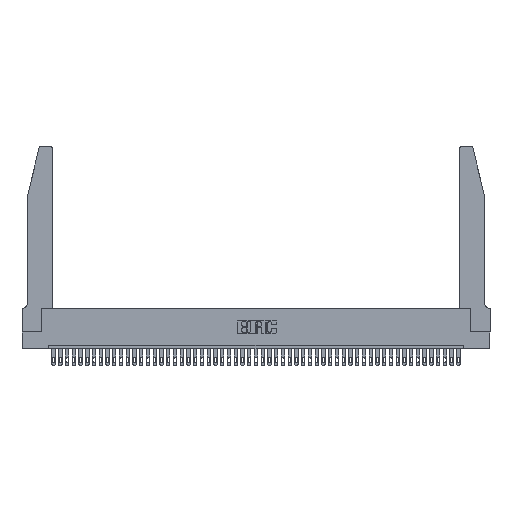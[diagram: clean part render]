
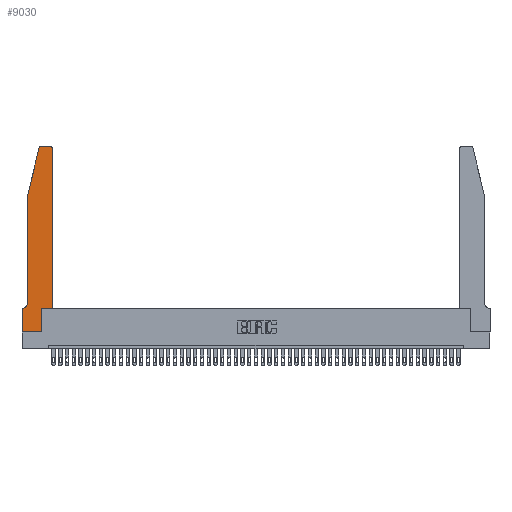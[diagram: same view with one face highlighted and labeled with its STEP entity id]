
A CAD part, top view. The second image highlights one B-rep face of the part: STEP entity #9030.
In plain terms, the highlighted planar face has unit normal (0, 0, 1).
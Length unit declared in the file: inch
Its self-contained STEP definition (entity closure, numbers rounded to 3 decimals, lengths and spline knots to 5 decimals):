
#95 = VERTEX_POINT ( 'NONE', #7106 ) ;
#144 = AXIS2_PLACEMENT_3D ( 'NONE', #27941, #35610, #2366 ) ;
#170 = ORIENTED_EDGE ( 'NONE', *, *, #24348, .T. ) ;
#1608 = DIRECTION ( 'NONE',  ( 0., 1., 0. ) ) ;
#2128 = CARTESIAN_POINT ( 'NONE',  ( 0.4205, 2.75, 0.37 ) ) ;
#2366 = DIRECTION ( 'NONE',  ( 1., 0., 0. ) ) ;
#3144 = VERTEX_POINT ( 'NONE', #28241 ) ;
#4175 = ORIENTED_EDGE ( 'NONE', *, *, #23835, .T. ) ;
#4460 = DIRECTION ( 'NONE',  ( -1., 0., 0. ) ) ;
#4820 = VERTEX_POINT ( 'NONE', #42210 ) ;
#4945 = VECTOR ( 'NONE', #26422, 39.37008 ) ;
#5229 = ORIENTED_EDGE ( 'NONE', *, *, #10144, .T. ) ;
#5287 = EDGE_CURVE ( 'NONE', #4820, #25033, #38751, .T. ) ;
#6729 = ORIENTED_EDGE ( 'NONE', *, *, #9586, .T. ) ;
#7106 = CARTESIAN_POINT ( 'NONE',  ( 0., 0.35, 0.37 ) ) ;
#7374 = LINE ( 'NONE', #19975, #15328 ) ;
#7543 = CIRCLE ( 'NONE', #144, 0.03 ) ;
#9030 = ADVANCED_FACE ( 'NONE', ( #33264 ), #16966, .T. ) ;
#9040 = DIRECTION ( 'NONE',  ( 1., 0., 0. ) ) ;
#9586 = EDGE_CURVE ( 'NONE', #3144, #27715, #7374, .T. ) ;
#10144 = EDGE_CURVE ( 'NONE', #19542, #3144, #37966, .T. ) ;
#10581 = CARTESIAN_POINT ( 'NONE',  ( 0.0755, 0.42, 0.37 ) ) ;
#11429 = VECTOR ( 'NONE', #36887, 39.37008 ) ;
#11593 = EDGE_CURVE ( 'NONE', #41714, #36071, #11748, .T. ) ;
#11667 = EDGE_CURVE ( 'NONE', #95, #19542, #26233, .T. ) ;
#11748 = LINE ( 'NONE', #12568, #47234 ) ;
#12568 = CARTESIAN_POINT ( 'NONE',  ( 0.4505, 0.35, 0.37 ) ) ;
#13299 = LINE ( 'NONE', #22866, #24337 ) ;
#13457 = DIRECTION ( 'NONE',  ( 1., 0., 0. ) ) ;
#13669 = CARTESIAN_POINT ( 'NONE',  ( 0.4505, 0.35, 0.37 ) ) ;
#13949 = EDGE_CURVE ( 'NONE', #34586, #14056, #14427, .T. ) ;
#14056 = VERTEX_POINT ( 'NONE', #46454 ) ;
#14427 = CIRCLE ( 'NONE', #47352, 0.07 ) ;
#14508 = CARTESIAN_POINT ( 'NONE',  ( 0.0055, 0.42, 0.37 ) ) ;
#14633 = VECTOR ( 'NONE', #15605, 39.37008 ) ;
#15246 = CARTESIAN_POINT ( 'NONE',  ( 0.0755, 2., 0.37 ) ) ;
#15328 = VECTOR ( 'NONE', #42264, 39.37008 ) ;
#15486 = CIRCLE ( 'NONE', #35171, 0.03 ) ;
#15596 = ORIENTED_EDGE ( 'NONE', *, *, #15885, .T. ) ;
#15605 = DIRECTION ( 'NONE',  ( 0., -1., 0. ) ) ;
#15843 = CARTESIAN_POINT ( 'NONE',  ( 0.4505, 2.72, 0.37 ) ) ;
#15885 = EDGE_CURVE ( 'NONE', #30623, #24158, #19601, .T. ) ;
#16187 = EDGE_CURVE ( 'NONE', #36071, #30623, #7543, .T. ) ;
#16415 = DIRECTION ( 'NONE',  ( -1., 0., 0. ) ) ;
#16966 = PLANE ( 'NONE',  #29522 ) ;
#18651 = DIRECTION ( 'NONE',  ( 0., 0., -1. ) ) ;
#19542 = VERTEX_POINT ( 'NONE', #23255 ) ;
#19601 = LINE ( 'NONE', #46045, #45235 ) ;
#19710 = ORIENTED_EDGE ( 'NONE', *, *, #32613, .T. ) ;
#19975 = CARTESIAN_POINT ( 'NONE',  ( 0.2865, 0.35, 0.37 ) ) ;
#20519 = ORIENTED_EDGE ( 'NONE', *, *, #5287, .T. ) ;
#20702 = CARTESIAN_POINT ( 'NONE',  ( 0., 0.35, 0.37 ) ) ;
#21926 = ORIENTED_EDGE ( 'NONE', *, *, #13949, .T. ) ;
#22655 = DIRECTION ( 'NONE',  ( 0., 0., 1. ) ) ;
#22698 = ORIENTED_EDGE ( 'NONE', *, *, #16187, .T. ) ;
#22866 = CARTESIAN_POINT ( 'NONE',  ( 0.0755, 0.35, 0.37 ) ) ;
#23255 = CARTESIAN_POINT ( 'NONE',  ( 0., 0., 0.37 ) ) ;
#23770 = CARTESIAN_POINT ( 'NONE',  ( 0., 0., 0.37 ) ) ;
#23835 = EDGE_CURVE ( 'NONE', #14056, #95, #13299, .T. ) ;
#24158 = VERTEX_POINT ( 'NONE', #37510 ) ;
#24337 = VECTOR ( 'NONE', #4460, 39.37008 ) ;
#24348 = EDGE_CURVE ( 'NONE', #24158, #4820, #15486, .T. ) ;
#24437 = CARTESIAN_POINT ( 'NONE',  ( 0.284, 2.72, 0.37 ) ) ;
#24560 = ORIENTED_EDGE ( 'NONE', *, *, #41828, .T. ) ;
#25033 = VERTEX_POINT ( 'NONE', #46265 ) ;
#26233 = LINE ( 'NONE', #23770, #14633 ) ;
#26422 = DIRECTION ( 'NONE',  ( 1., 0., 0. ) ) ;
#27062 = ORIENTED_EDGE ( 'NONE', *, *, #11593, .T. ) ;
#27235 = LINE ( 'NONE', #15246, #38295 ) ;
#27715 = VERTEX_POINT ( 'NONE', #45758 ) ;
#27765 = CARTESIAN_POINT ( 'NONE',  ( 0.4505, 0.35, 0.37 ) ) ;
#27941 = CARTESIAN_POINT ( 'NONE',  ( 0.4205, 2.72, 0.37 ) ) ;
#28241 = CARTESIAN_POINT ( 'NONE',  ( 0.2865, 0., 0.37 ) ) ;
#29522 = AXIS2_PLACEMENT_3D ( 'NONE', #20702, #46759, #13457 ) ;
#30623 = VERTEX_POINT ( 'NONE', #2128 ) ;
#32613 = EDGE_CURVE ( 'NONE', #25033, #34586, #27235, .T. ) ;
#33264 = FACE_OUTER_BOUND ( 'NONE', #44876, .T. ) ;
#33842 = DIRECTION ( 'NONE',  ( -1., 0., 0. ) ) ;
#34297 = DIRECTION ( 'NONE',  ( 0., -1., 0. ) ) ;
#34586 = VERTEX_POINT ( 'NONE', #10581 ) ;
#34765 = VECTOR ( 'NONE', #39327, 39.37008 ) ;
#35171 = AXIS2_PLACEMENT_3D ( 'NONE', #24437, #22655, #9040 ) ;
#35610 = DIRECTION ( 'NONE',  ( 0., 0., 1. ) ) ;
#35949 = LINE ( 'NONE', #13669, #34765 ) ;
#36071 = VERTEX_POINT ( 'NONE', #15843 ) ;
#36887 = DIRECTION ( 'NONE',  ( -0.239, -0.971, 0. ) ) ;
#37510 = CARTESIAN_POINT ( 'NONE',  ( 0.284, 2.75, 0.37 ) ) ;
#37966 = LINE ( 'NONE', #44036, #4945 ) ;
#38295 = VECTOR ( 'NONE', #34297, 39.37008 ) ;
#38751 = LINE ( 'NONE', #40310, #11429 ) ;
#39327 = DIRECTION ( 'NONE',  ( 1., 0., 0. ) ) ;
#40310 = CARTESIAN_POINT ( 'NONE',  ( 0.0755, 2., 0.37 ) ) ;
#41714 = VERTEX_POINT ( 'NONE', #27765 ) ;
#41828 = EDGE_CURVE ( 'NONE', #27715, #41714, #35949, .T. ) ;
#42210 = CARTESIAN_POINT ( 'NONE',  ( 0.25487, 2.72718, 0.37 ) ) ;
#42264 = DIRECTION ( 'NONE',  ( 0., 1., 0. ) ) ;
#42399 = ORIENTED_EDGE ( 'NONE', *, *, #11667, .T. ) ;
#44036 = CARTESIAN_POINT ( 'NONE',  ( 0., 0., 0.37 ) ) ;
#44876 = EDGE_LOOP ( 'NONE', ( #15596, #170, #20519, #19710, #21926, #4175, #42399, #5229, #6729, #24560, #27062, #22698 ) ) ;
#45235 = VECTOR ( 'NONE', #16415, 39.37008 ) ;
#45758 = CARTESIAN_POINT ( 'NONE',  ( 0.2865, 0.35, 0.37 ) ) ;
#46045 = CARTESIAN_POINT ( 'NONE',  ( 0.2605, 2.75, 0.37 ) ) ;
#46265 = CARTESIAN_POINT ( 'NONE',  ( 0.0755, 2., 0.37 ) ) ;
#46454 = CARTESIAN_POINT ( 'NONE',  ( 0.0055, 0.35, 0.37 ) ) ;
#46759 = DIRECTION ( 'NONE',  ( 0., 0., 1. ) ) ;
#47234 = VECTOR ( 'NONE', #1608, 39.37008 ) ;
#47352 = AXIS2_PLACEMENT_3D ( 'NONE', #14508, #18651, #33842 ) ;
